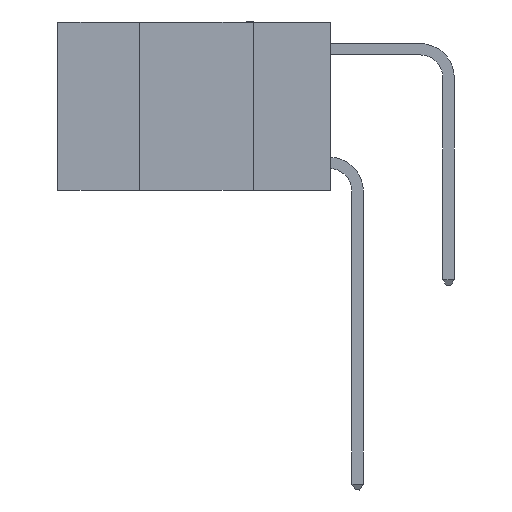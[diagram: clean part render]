
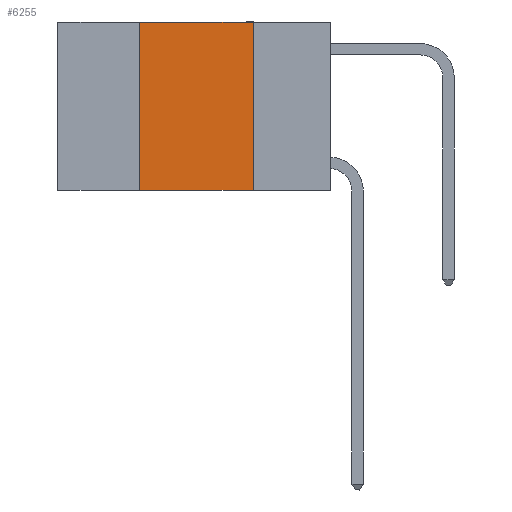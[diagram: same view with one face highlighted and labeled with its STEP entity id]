
A CAD part, left-side view. The second image highlights one B-rep face of the part: STEP entity #6255.
In plain terms, the highlighted planar face has unit normal (-1, 0, 0).
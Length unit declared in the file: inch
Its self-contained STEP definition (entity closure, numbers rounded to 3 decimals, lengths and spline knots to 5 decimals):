
#1263 = CARTESIAN_POINT ( 'NONE',  ( 0., 0.42, 0. ) ) ;
#1624 = LINE ( 'NONE', #21808, #21039 ) ;
#1880 = AXIS2_PLACEMENT_3D ( 'NONE', #29523, #9847, #26934 ) ;
#2531 = VECTOR ( 'NONE', #12041, 39.37008 ) ;
#2571 = PLANE ( 'NONE',  #1880 ) ;
#5837 = DIRECTION ( 'NONE',  ( 0., 0., 1. ) ) ;
#6015 = VERTEX_POINT ( 'NONE', #12310 ) ;
#6255 = ADVANCED_FACE ( 'NONE', ( #26623 ), #2571, .F. ) ;
#6324 = ORIENTED_EDGE ( 'NONE', *, *, #20046, .T. ) ;
#7109 = VECTOR ( 'NONE', #5837, 39.37008 ) ;
#7940 = CARTESIAN_POINT ( 'NONE',  ( 0., 0.17, 0. ) ) ;
#9847 = DIRECTION ( 'NONE',  ( 1., 0., 0. ) ) ;
#10671 = LINE ( 'NONE', #20490, #7109 ) ;
#11800 = VERTEX_POINT ( 'NONE', #1263 ) ;
#12041 = DIRECTION ( 'NONE',  ( 0., -1., 0. ) ) ;
#12310 = CARTESIAN_POINT ( 'NONE',  ( 0., 0.42, -0.37 ) ) ;
#13666 = ORIENTED_EDGE ( 'NONE', *, *, #19084, .F. ) ;
#14097 = EDGE_LOOP ( 'NONE', ( #20688, #27532, #13666, #6324 ) ) ;
#14508 = CARTESIAN_POINT ( 'NONE',  ( 0., 0.17, -0.37 ) ) ;
#15358 = LINE ( 'NONE', #7940, #27861 ) ;
#19084 = EDGE_CURVE ( 'NONE', #6015, #11800, #10671, .T. ) ;
#19620 = LINE ( 'NONE', #23998, #2531 ) ;
#20046 = EDGE_CURVE ( 'NONE', #6015, #22942, #1624, .T. ) ;
#20418 = EDGE_CURVE ( 'NONE', #11800, #20512, #19620, .T. ) ;
#20490 = CARTESIAN_POINT ( 'NONE',  ( 0., 0.42, 0. ) ) ;
#20512 = VERTEX_POINT ( 'NONE', #26407 ) ;
#20688 = ORIENTED_EDGE ( 'NONE', *, *, #22709, .F. ) ;
#21039 = VECTOR ( 'NONE', #26160, 39.37008 ) ;
#21808 = CARTESIAN_POINT ( 'NONE',  ( 0., 0.6, -0.37 ) ) ;
#22709 = EDGE_CURVE ( 'NONE', #20512, #22942, #15358, .T. ) ;
#22942 = VERTEX_POINT ( 'NONE', #14508 ) ;
#23998 = CARTESIAN_POINT ( 'NONE',  ( 0., 0.6, 0. ) ) ;
#25020 = DIRECTION ( 'NONE',  ( 0., 0., -1. ) ) ;
#26160 = DIRECTION ( 'NONE',  ( 0., -1., 0. ) ) ;
#26407 = CARTESIAN_POINT ( 'NONE',  ( 0., 0.17, 0. ) ) ;
#26623 = FACE_OUTER_BOUND ( 'NONE', #14097, .T. ) ;
#26934 = DIRECTION ( 'NONE',  ( 0., 0., -1. ) ) ;
#27532 = ORIENTED_EDGE ( 'NONE', *, *, #20418, .F. ) ;
#27861 = VECTOR ( 'NONE', #25020, 39.37008 ) ;
#29523 = CARTESIAN_POINT ( 'NONE',  ( 0., 0.6, 0. ) ) ;
